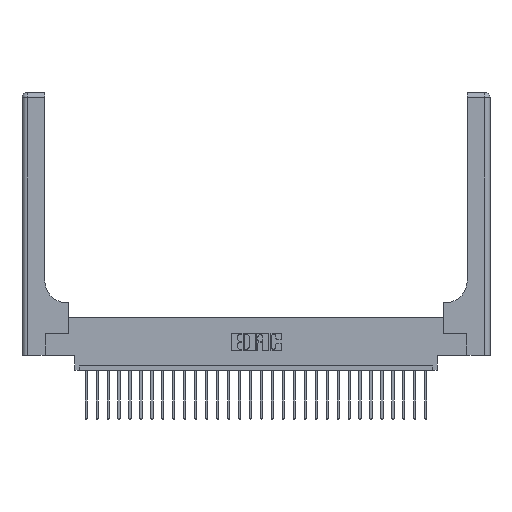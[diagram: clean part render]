
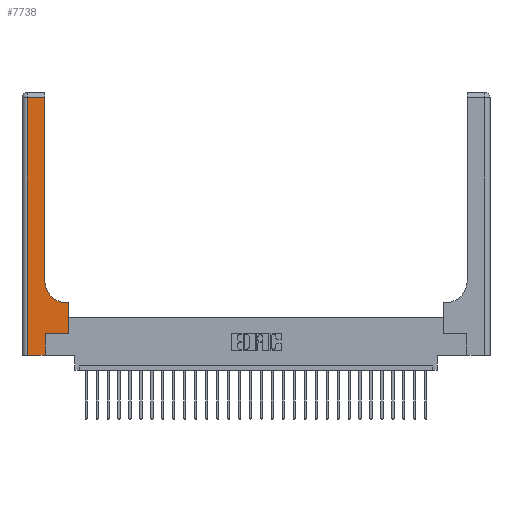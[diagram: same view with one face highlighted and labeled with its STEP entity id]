
A CAD part, top view. The second image highlights one B-rep face of the part: STEP entity #7738.
In plain terms, the highlighted planar face has unit normal (0, 0, 1).
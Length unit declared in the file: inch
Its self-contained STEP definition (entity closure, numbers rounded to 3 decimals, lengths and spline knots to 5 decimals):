
#131 = VECTOR ( 'NONE', #11019, 39.37008 ) ;
#436 = LINE ( 'NONE', #4631, #131 ) ;
#1238 = VERTEX_POINT ( 'NONE', #9384 ) ;
#2220 = CARTESIAN_POINT ( 'NONE',  ( 0.528, 0.25, 0.37 ) ) ;
#2224 = VECTOR ( 'NONE', #11034, 39.37008 ) ;
#3204 = VERTEX_POINT ( 'NONE', #26159 ) ;
#3909 = VECTOR ( 'NONE', #4860, 39.37008 ) ;
#4631 = CARTESIAN_POINT ( 'NONE',  ( 0.06, 3., 0.37 ) ) ;
#4787 = CARTESIAN_POINT ( 'NONE',  ( 0.06, 2.94, 0.37 ) ) ;
#4860 = DIRECTION ( 'NONE',  ( -1., 0., 0. ) ) ;
#4986 = VECTOR ( 'NONE', #18308, 39.37008 ) ;
#5068 = LINE ( 'NONE', #15426, #12979 ) ;
#5250 = CARTESIAN_POINT ( 'NONE',  ( 0., 3., 0.37 ) ) ;
#5372 = DIRECTION ( 'NONE',  ( -1., 0., 0. ) ) ;
#5648 = DIRECTION ( 'NONE',  ( 0., 0., -1. ) ) ;
#7159 = CARTESIAN_POINT ( 'NONE',  ( 0.26, 2.94, 0.37 ) ) ;
#7319 = VECTOR ( 'NONE', #19667, 39.37008 ) ;
#7616 = DIRECTION ( 'NONE',  ( 1., 0., 0. ) ) ;
#7738 = ADVANCED_FACE ( 'NONE', ( #9057 ), #8514, .F. ) ;
#8456 = CARTESIAN_POINT ( 'NONE',  ( 0., 0., 0.37 ) ) ;
#8514 = PLANE ( 'NONE',  #18880 ) ;
#9057 = FACE_OUTER_BOUND ( 'NONE', #9358, .T. ) ;
#9143 = LINE ( 'NONE', #13765, #2224 ) ;
#9164 = LINE ( 'NONE', #26105, #7319 ) ;
#9358 = EDGE_LOOP ( 'NONE', ( #26127, #21953, #10970, #26685, #25299, #16578, #22566, #16812, #26371 ) ) ;
#9384 = CARTESIAN_POINT ( 'NONE',  ( 0.265, 0.25, 0.37 ) ) ;
#10539 = CARTESIAN_POINT ( 'NONE',  ( 0.528, 0.25, 0.37 ) ) ;
#10878 = EDGE_CURVE ( 'NONE', #18362, #11265, #436, .T. ) ;
#10902 = VERTEX_POINT ( 'NONE', #14988 ) ;
#10970 = ORIENTED_EDGE ( 'NONE', *, *, #10878, .T. ) ;
#11019 = DIRECTION ( 'NONE',  ( 0., -1., 0. ) ) ;
#11034 = DIRECTION ( 'NONE',  ( -1., 0., 0. ) ) ;
#11265 = VERTEX_POINT ( 'NONE', #14683 ) ;
#11405 = VERTEX_POINT ( 'NONE', #7159 ) ;
#11478 = CARTESIAN_POINT ( 'NONE',  ( 0.265, 0.25, 0.37 ) ) ;
#11503 = VECTOR ( 'NONE', #20639, 39.37008 ) ;
#11615 = LINE ( 'NONE', #11478, #12394 ) ;
#12394 = VECTOR ( 'NONE', #13946, 39.37008 ) ;
#12802 = AXIS2_PLACEMENT_3D ( 'NONE', #17720, #25811, #7616 ) ;
#12979 = VECTOR ( 'NONE', #17741, 39.37008 ) ;
#13413 = EDGE_CURVE ( 'NONE', #25481, #11405, #9164, .T. ) ;
#13470 = EDGE_CURVE ( 'NONE', #3204, #1238, #5068, .T. ) ;
#13765 = CARTESIAN_POINT ( 'NONE',  ( 0.26, 0.6, 0.37 ) ) ;
#13946 = DIRECTION ( 'NONE',  ( 1., 0., 0. ) ) ;
#14022 = EDGE_CURVE ( 'NONE', #11405, #18362, #15763, .T. ) ;
#14683 = CARTESIAN_POINT ( 'NONE',  ( 0.06, 0., 0.37 ) ) ;
#14973 = CIRCLE ( 'NONE', #12802, 0.25 ) ;
#14988 = CARTESIAN_POINT ( 'NONE',  ( 0.51, 0.6, 0.37 ) ) ;
#15426 = CARTESIAN_POINT ( 'NONE',  ( 0.265, 0., 0.37 ) ) ;
#15510 = CARTESIAN_POINT ( 'NONE',  ( 0.26, 0.85, 0.37 ) ) ;
#15763 = LINE ( 'NONE', #26167, #3909 ) ;
#16377 = LINE ( 'NONE', #8456, #4986 ) ;
#16578 = ORIENTED_EDGE ( 'NONE', *, *, #23357, .T. ) ;
#16812 = ORIENTED_EDGE ( 'NONE', *, *, #19635, .T. ) ;
#17720 = CARTESIAN_POINT ( 'NONE',  ( 0.51, 0.85, 0.37 ) ) ;
#17741 = DIRECTION ( 'NONE',  ( 0., 1., 0. ) ) ;
#18308 = DIRECTION ( 'NONE',  ( 1., 0., 0. ) ) ;
#18362 = VERTEX_POINT ( 'NONE', #4787 ) ;
#18734 = CARTESIAN_POINT ( 'NONE',  ( 0.528, 0.6, 0.37 ) ) ;
#18880 = AXIS2_PLACEMENT_3D ( 'NONE', #5250, #5648, #5372 ) ;
#18928 = VERTEX_POINT ( 'NONE', #18734 ) ;
#19635 = EDGE_CURVE ( 'NONE', #18928, #10902, #9143, .T. ) ;
#19667 = DIRECTION ( 'NONE',  ( 0., 1., 0. ) ) ;
#20639 = DIRECTION ( 'NONE',  ( 0., 1., 0. ) ) ;
#20850 = EDGE_CURVE ( 'NONE', #10902, #25481, #14973, .T. ) ;
#21953 = ORIENTED_EDGE ( 'NONE', *, *, #14022, .T. ) ;
#22566 = ORIENTED_EDGE ( 'NONE', *, *, #23107, .T. ) ;
#23107 = EDGE_CURVE ( 'NONE', #26007, #18928, #26692, .T. ) ;
#23357 = EDGE_CURVE ( 'NONE', #1238, #26007, #11615, .T. ) ;
#23582 = EDGE_CURVE ( 'NONE', #11265, #3204, #16377, .T. ) ;
#25299 = ORIENTED_EDGE ( 'NONE', *, *, #13470, .T. ) ;
#25481 = VERTEX_POINT ( 'NONE', #15510 ) ;
#25811 = DIRECTION ( 'NONE',  ( 0., 0., -1. ) ) ;
#26007 = VERTEX_POINT ( 'NONE', #2220 ) ;
#26105 = CARTESIAN_POINT ( 'NONE',  ( 0.26, 3., 0.37 ) ) ;
#26127 = ORIENTED_EDGE ( 'NONE', *, *, #13413, .T. ) ;
#26159 = CARTESIAN_POINT ( 'NONE',  ( 0.265, 0., 0.37 ) ) ;
#26167 = CARTESIAN_POINT ( 'NONE',  ( 0., 2.94, 0.37 ) ) ;
#26371 = ORIENTED_EDGE ( 'NONE', *, *, #20850, .T. ) ;
#26685 = ORIENTED_EDGE ( 'NONE', *, *, #23582, .T. ) ;
#26692 = LINE ( 'NONE', #10539, #11503 ) ;
